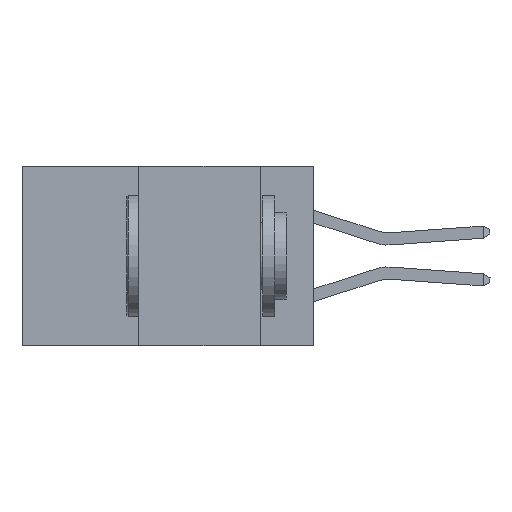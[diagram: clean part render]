
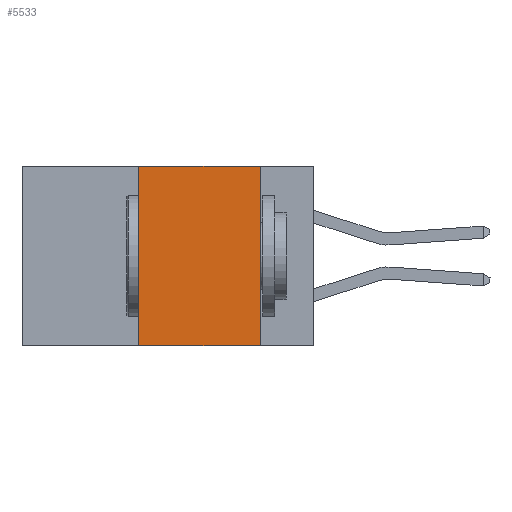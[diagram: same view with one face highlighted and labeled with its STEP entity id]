
A CAD part, left-side view. The second image highlights one B-rep face of the part: STEP entity #5533.
In plain terms, the highlighted planar face has unit normal (-1, 0, 0).
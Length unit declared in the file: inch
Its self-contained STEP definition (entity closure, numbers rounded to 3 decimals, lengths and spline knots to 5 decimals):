
#682 = DIRECTION ( 'NONE',  ( 1., 0., 0. ) ) ;
#773 = PLANE ( 'NONE',  #28857 ) ;
#1013 = CARTESIAN_POINT ( 'NONE',  ( 0., 0.36, 0. ) ) ;
#1631 = FACE_OUTER_BOUND ( 'NONE', #12407, .T. ) ;
#1881 = ORIENTED_EDGE ( 'NONE', *, *, #3196, .T. ) ;
#2044 = DIRECTION ( 'NONE',  ( 0., -1., 0. ) ) ;
#2713 = VERTEX_POINT ( 'NONE', #24154 ) ;
#3196 = EDGE_CURVE ( 'NONE', #23681, #8943, #17630, .T. ) ;
#4488 = VECTOR ( 'NONE', #30944, 39.37008 ) ;
#4655 = CARTESIAN_POINT ( 'NONE',  ( 0., 0.6, 0. ) ) ;
#5223 = VERTEX_POINT ( 'NONE', #14178 ) ;
#5533 = ADVANCED_FACE ( 'NONE', ( #1631 ), #773, .F. ) ;
#6822 = CARTESIAN_POINT ( 'NONE',  ( 0., 0.6, -0.37 ) ) ;
#8943 = VERTEX_POINT ( 'NONE', #23291 ) ;
#10838 = CARTESIAN_POINT ( 'NONE',  ( 0., 0.11, 0. ) ) ;
#12407 = EDGE_LOOP ( 'NONE', ( #25239, #28691, #14315, #1881 ) ) ;
#14178 = CARTESIAN_POINT ( 'NONE',  ( 0., 0.36, 0. ) ) ;
#14315 = ORIENTED_EDGE ( 'NONE', *, *, #18712, .F. ) ;
#16984 = EDGE_CURVE ( 'NONE', #5223, #2713, #27468, .T. ) ;
#17586 = CARTESIAN_POINT ( 'NONE',  ( 0., 0.36, -0.37 ) ) ;
#17630 = LINE ( 'NONE', #6822, #4488 ) ;
#18109 = VECTOR ( 'NONE', #23030, 39.37008 ) ;
#18712 = EDGE_CURVE ( 'NONE', #23681, #5223, #26573, .T. ) ;
#19921 = LINE ( 'NONE', #10838, #25726 ) ;
#20508 = DIRECTION ( 'NONE',  ( 0., 0., -1. ) ) ;
#23030 = DIRECTION ( 'NONE',  ( 0., 0., 1. ) ) ;
#23291 = CARTESIAN_POINT ( 'NONE',  ( 0., 0.11, -0.37 ) ) ;
#23681 = VERTEX_POINT ( 'NONE', #17586 ) ;
#24154 = CARTESIAN_POINT ( 'NONE',  ( 0., 0.11, 0. ) ) ;
#25239 = ORIENTED_EDGE ( 'NONE', *, *, #28714, .F. ) ;
#25726 = VECTOR ( 'NONE', #28049, 39.37008 ) ;
#26573 = LINE ( 'NONE', #1013, #18109 ) ;
#27468 = LINE ( 'NONE', #4655, #29783 ) ;
#28049 = DIRECTION ( 'NONE',  ( 0., 0., -1. ) ) ;
#28691 = ORIENTED_EDGE ( 'NONE', *, *, #16984, .F. ) ;
#28714 = EDGE_CURVE ( 'NONE', #2713, #8943, #19921, .T. ) ;
#28857 = AXIS2_PLACEMENT_3D ( 'NONE', #29990, #682, #20508 ) ;
#29783 = VECTOR ( 'NONE', #2044, 39.37008 ) ;
#29990 = CARTESIAN_POINT ( 'NONE',  ( 0., 0.6, 0. ) ) ;
#30944 = DIRECTION ( 'NONE',  ( 0., -1., 0. ) ) ;
